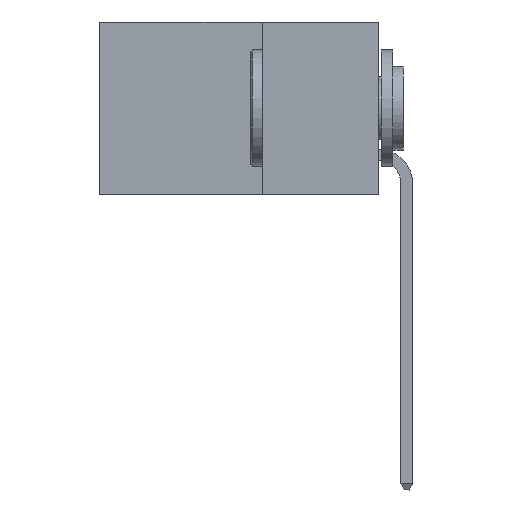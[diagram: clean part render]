
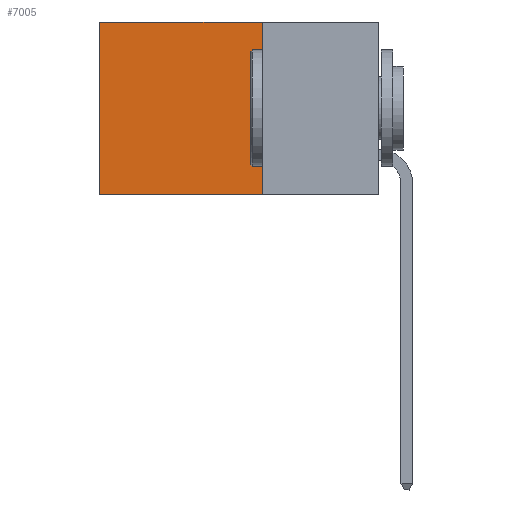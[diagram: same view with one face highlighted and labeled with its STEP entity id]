
A CAD part, left-side view. The second image highlights one B-rep face of the part: STEP entity #7005.
In plain terms, the highlighted planar face has unit normal (-1, 0, 0).
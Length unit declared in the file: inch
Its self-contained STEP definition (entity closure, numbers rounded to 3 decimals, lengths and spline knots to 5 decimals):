
#149 = AXIS2_PLACEMENT_3D ( 'NONE', #10312, #3001, #324 ) ;
#324 = DIRECTION ( 'NONE',  ( 0., 0., -1. ) ) ;
#588 = LINE ( 'NONE', #724, #1163 ) ;
#724 = CARTESIAN_POINT ( 'NONE',  ( 0.298, 0.25, -0.37 ) ) ;
#852 = CARTESIAN_POINT ( 'NONE',  ( 0.298, 0.6, 0. ) ) ;
#971 = ORIENTED_EDGE ( 'NONE', *, *, #3746, .F. ) ;
#1163 = VECTOR ( 'NONE', #7953, 39.37008 ) ;
#1176 = EDGE_LOOP ( 'NONE', ( #3678, #6969, #971, #11054 ) ) ;
#1343 = LINE ( 'NONE', #852, #7409 ) ;
#2091 = PLANE ( 'NONE',  #149 ) ;
#2283 = VERTEX_POINT ( 'NONE', #2656 ) ;
#2656 = CARTESIAN_POINT ( 'NONE',  ( 0.298, 0.25, -0.37 ) ) ;
#2751 = FACE_OUTER_BOUND ( 'NONE', #1176, .T. ) ;
#3001 = DIRECTION ( 'NONE',  ( 1., 0., 0. ) ) ;
#3454 = DIRECTION ( 'NONE',  ( 0., 0., -1. ) ) ;
#3678 = ORIENTED_EDGE ( 'NONE', *, *, #8039, .T. ) ;
#3694 = VERTEX_POINT ( 'NONE', #7540 ) ;
#3746 = EDGE_CURVE ( 'NONE', #3694, #2283, #5328, .T. ) ;
#3927 = DIRECTION ( 'NONE',  ( 0., 1., 0. ) ) ;
#4767 = VERTEX_POINT ( 'NONE', #11386 ) ;
#5328 = LINE ( 'NONE', #6722, #8034 ) ;
#5621 = LINE ( 'NONE', #5727, #7908 ) ;
#5727 = CARTESIAN_POINT ( 'NONE',  ( 0.298, 0.25, 0. ) ) ;
#6722 = CARTESIAN_POINT ( 'NONE',  ( 0.298, 0.25, 0. ) ) ;
#6969 = ORIENTED_EDGE ( 'NONE', *, *, #9122, .F. ) ;
#7005 = ADVANCED_FACE ( 'NONE', ( #2751 ), #2091, .F. ) ;
#7409 = VECTOR ( 'NONE', #3454, 39.37008 ) ;
#7540 = CARTESIAN_POINT ( 'NONE',  ( 0.298, 0.25, 0. ) ) ;
#7908 = VECTOR ( 'NONE', #3927, 39.37008 ) ;
#7953 = DIRECTION ( 'NONE',  ( 0., 1., 0. ) ) ;
#8034 = VECTOR ( 'NONE', #9454, 39.37008 ) ;
#8039 = EDGE_CURVE ( 'NONE', #4767, #11666, #1343, .T. ) ;
#9122 = EDGE_CURVE ( 'NONE', #2283, #11666, #588, .T. ) ;
#9454 = DIRECTION ( 'NONE',  ( 0., 0., -1. ) ) ;
#10213 = EDGE_CURVE ( 'NONE', #3694, #4767, #5621, .T. ) ;
#10312 = CARTESIAN_POINT ( 'NONE',  ( 0.298, 0.25, 0. ) ) ;
#11054 = ORIENTED_EDGE ( 'NONE', *, *, #10213, .T. ) ;
#11386 = CARTESIAN_POINT ( 'NONE',  ( 0.298, 0.6, 0. ) ) ;
#11552 = CARTESIAN_POINT ( 'NONE',  ( 0.298, 0.6, -0.37 ) ) ;
#11666 = VERTEX_POINT ( 'NONE', #11552 ) ;
